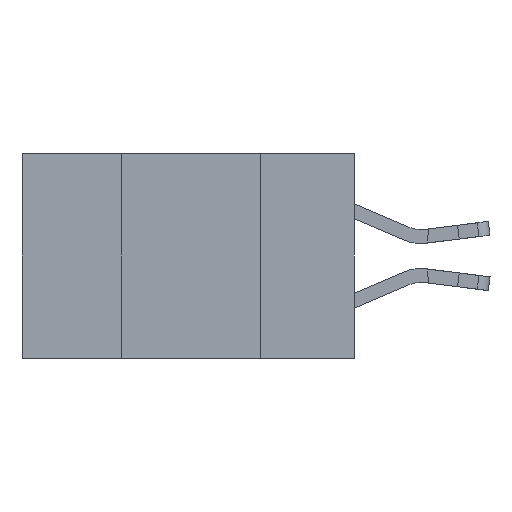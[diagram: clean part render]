
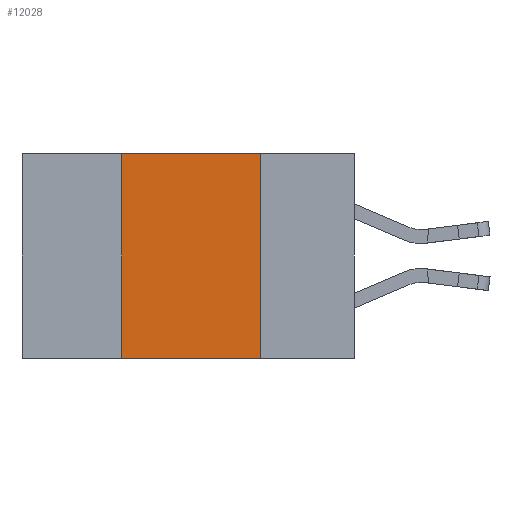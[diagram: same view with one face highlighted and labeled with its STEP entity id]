
A CAD part, left-side view. The second image highlights one B-rep face of the part: STEP entity #12028.
In plain terms, the highlighted planar face has unit normal (-1, 0, 0).
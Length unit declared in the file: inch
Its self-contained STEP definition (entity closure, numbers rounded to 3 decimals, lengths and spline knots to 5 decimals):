
#222 = LINE ( 'NONE', #8578, #23122 ) ;
#1383 = DIRECTION ( 'NONE',  ( 0., 0., 1. ) ) ;
#1674 = ORIENTED_EDGE ( 'NONE', *, *, #13937, .T. ) ;
#2436 = VERTEX_POINT ( 'NONE', #19869 ) ;
#3418 = LINE ( 'NONE', #8874, #7802 ) ;
#4891 = EDGE_CURVE ( 'NONE', #2436, #18556, #222, .T. ) ;
#5849 = AXIS2_PLACEMENT_3D ( 'NONE', #14630, #12743, #12918 ) ;
#7168 = VECTOR ( 'NONE', #11443, 39.37008 ) ;
#7802 = VECTOR ( 'NONE', #14331, 39.37008 ) ;
#8578 = CARTESIAN_POINT ( 'NONE',  ( 0., 0.6, 0. ) ) ;
#8864 = DIRECTION ( 'NONE',  ( 0., -1., 0. ) ) ;
#8874 = CARTESIAN_POINT ( 'NONE',  ( 0., 0.6, -0.37 ) ) ;
#9266 = PLANE ( 'NONE',  #5849 ) ;
#9772 = VERTEX_POINT ( 'NONE', #20783 ) ;
#10400 = ORIENTED_EDGE ( 'NONE', *, *, #14832, .F. ) ;
#10615 = EDGE_LOOP ( 'NONE', ( #10400, #19847, #20399, #1674 ) ) ;
#11443 = DIRECTION ( 'NONE',  ( 0., 0., -1. ) ) ;
#11452 = FACE_OUTER_BOUND ( 'NONE', #10615, .T. ) ;
#12028 = ADVANCED_FACE ( 'NONE', ( #11452 ), #9266, .F. ) ;
#12743 = DIRECTION ( 'NONE',  ( 1., 0., 0. ) ) ;
#12918 = DIRECTION ( 'NONE',  ( 0., 0., -1. ) ) ;
#13446 = VECTOR ( 'NONE', #1383, 39.37008 ) ;
#13937 = EDGE_CURVE ( 'NONE', #13947, #9772, #3418, .T. ) ;
#13947 = VERTEX_POINT ( 'NONE', #16168 ) ;
#14002 = LINE ( 'NONE', #21261, #13446 ) ;
#14331 = DIRECTION ( 'NONE',  ( 0., -1., 0. ) ) ;
#14630 = CARTESIAN_POINT ( 'NONE',  ( 0., 0.6, 0. ) ) ;
#14832 = EDGE_CURVE ( 'NONE', #18556, #9772, #15617, .T. ) ;
#15617 = LINE ( 'NONE', #22035, #7168 ) ;
#16168 = CARTESIAN_POINT ( 'NONE',  ( 0., 0.42, -0.37 ) ) ;
#18446 = CARTESIAN_POINT ( 'NONE',  ( 0., 0.17, 0. ) ) ;
#18556 = VERTEX_POINT ( 'NONE', #18446 ) ;
#19847 = ORIENTED_EDGE ( 'NONE', *, *, #4891, .F. ) ;
#19869 = CARTESIAN_POINT ( 'NONE',  ( 0., 0.42, 0. ) ) ;
#20399 = ORIENTED_EDGE ( 'NONE', *, *, #21447, .F. ) ;
#20783 = CARTESIAN_POINT ( 'NONE',  ( 0., 0.17, -0.37 ) ) ;
#21261 = CARTESIAN_POINT ( 'NONE',  ( 0., 0.42, -0.37 ) ) ;
#21447 = EDGE_CURVE ( 'NONE', #13947, #2436, #14002, .T. ) ;
#22035 = CARTESIAN_POINT ( 'NONE',  ( 0., 0.17, -0.37 ) ) ;
#23122 = VECTOR ( 'NONE', #8864, 39.37008 ) ;
